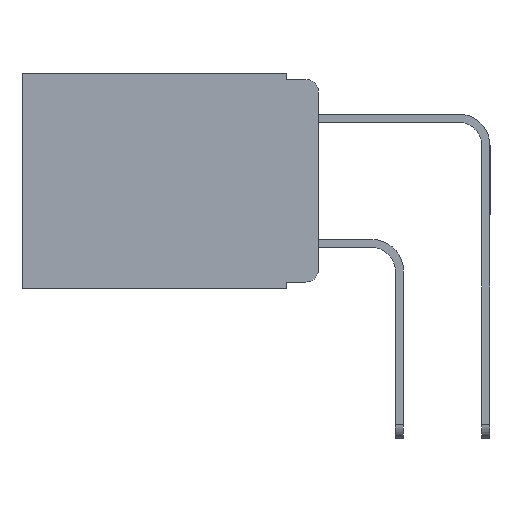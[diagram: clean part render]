
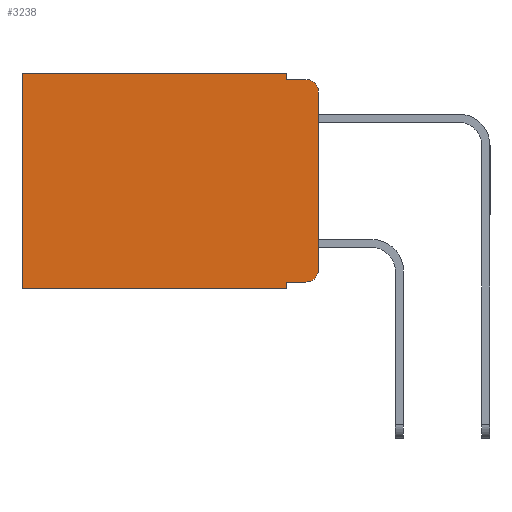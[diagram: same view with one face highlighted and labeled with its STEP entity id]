
A CAD part, left-side view. The second image highlights one B-rep face of the part: STEP entity #3238.
In plain terms, the highlighted planar face has unit normal (-1, 0, 0).
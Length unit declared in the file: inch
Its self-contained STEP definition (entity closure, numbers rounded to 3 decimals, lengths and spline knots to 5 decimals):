
#188 = ORIENTED_EDGE ( 'NONE', *, *, #21089, .T. ) ;
#479 = VECTOR ( 'NONE', #4422, 39.37008 ) ;
#505 = DIRECTION ( 'NONE',  ( 0., 0., -1. ) ) ;
#839 = DIRECTION ( 'NONE',  ( -1., 0., 0. ) ) ;
#938 = CARTESIAN_POINT ( 'NONE',  ( 0.298, 0.473, 0. ) ) ;
#1223 = CARTESIAN_POINT ( 'NONE',  ( 0.298, 0.051, 0. ) ) ;
#1309 = CARTESIAN_POINT ( 'NONE',  ( 0.298, 0.051, 0. ) ) ;
#1389 = CIRCLE ( 'NONE', #4869, 0.02 ) ;
#1470 = LINE ( 'NONE', #21075, #6059 ) ;
#1650 = LINE ( 'NONE', #11820, #15034 ) ;
#1971 = EDGE_CURVE ( 'NONE', #16292, #12738, #1470, .T. ) ;
#1996 = VERTEX_POINT ( 'NONE', #11594 ) ;
#2025 = VECTOR ( 'NONE', #15394, 39.37008 ) ;
#2137 = CARTESIAN_POINT ( 'NONE',  ( 0.298, 0.02, -0.01 ) ) ;
#2178 = CARTESIAN_POINT ( 'NONE',  ( 0.298, 0.051, 0. ) ) ;
#2614 = LINE ( 'NONE', #1223, #11169 ) ;
#2741 = ORIENTED_EDGE ( 'NONE', *, *, #18984, .F. ) ;
#2787 = DIRECTION ( 'NONE',  ( -1., 0., 0. ) ) ;
#2960 = DIRECTION ( 'NONE',  ( 0., 0., -1. ) ) ;
#3118 = DIRECTION ( 'NONE',  ( 0., 0., -1. ) ) ;
#3238 = ADVANCED_FACE ( 'NONE', ( #14812 ), #8622, .F. ) ;
#3830 = EDGE_CURVE ( 'NONE', #15052, #7431, #17042, .T. ) ;
#4422 = DIRECTION ( 'NONE',  ( 0., 0., -1. ) ) ;
#4861 = VERTEX_POINT ( 'NONE', #8842 ) ;
#4869 = AXIS2_PLACEMENT_3D ( 'NONE', #12919, #2787, #14503 ) ;
#5413 = CARTESIAN_POINT ( 'NONE',  ( 0.298, 0., 0. ) ) ;
#5426 = ORIENTED_EDGE ( 'NONE', *, *, #17950, .T. ) ;
#6059 = VECTOR ( 'NONE', #3118, 39.37008 ) ;
#6281 = CARTESIAN_POINT ( 'NONE',  ( 0.298, 0., -0.03 ) ) ;
#6320 = VERTEX_POINT ( 'NONE', #18817 ) ;
#7232 = DIRECTION ( 'NONE',  ( 0., 1., 0. ) ) ;
#7431 = VERTEX_POINT ( 'NONE', #15783 ) ;
#7881 = VERTEX_POINT ( 'NONE', #2137 ) ;
#7952 = VECTOR ( 'NONE', #17075, 39.37008 ) ;
#8490 = VERTEX_POINT ( 'NONE', #17010 ) ;
#8622 = PLANE ( 'NONE',  #13814 ) ;
#8842 = CARTESIAN_POINT ( 'NONE',  ( 0.298, 0.02, -0.333 ) ) ;
#8873 = ORIENTED_EDGE ( 'NONE', *, *, #16742, .T. ) ;
#9361 = ORIENTED_EDGE ( 'NONE', *, *, #14760, .T. ) ;
#10233 = CARTESIAN_POINT ( 'NONE',  ( 0.298, 0.051, -0.343 ) ) ;
#10744 = VECTOR ( 'NONE', #7232, 39.37008 ) ;
#11110 = CARTESIAN_POINT ( 'NONE',  ( 0.298, 0.02, -0.03 ) ) ;
#11169 = VECTOR ( 'NONE', #2960, 39.37008 ) ;
#11594 = CARTESIAN_POINT ( 'NONE',  ( 0.298, 0.473, 0. ) ) ;
#11820 = CARTESIAN_POINT ( 'NONE',  ( 0.298, 0.051, -0.333 ) ) ;
#11885 = DIRECTION ( 'NONE',  ( 0., 0., -1. ) ) ;
#12180 = CARTESIAN_POINT ( 'NONE',  ( 0.298, 0., -0.313 ) ) ;
#12728 = DIRECTION ( 'NONE',  ( 0., 0., -1. ) ) ;
#12738 = VERTEX_POINT ( 'NONE', #12180 ) ;
#12799 = AXIS2_PLACEMENT_3D ( 'NONE', #11110, #839, #12728 ) ;
#12919 = CARTESIAN_POINT ( 'NONE',  ( 0.298, 0.02, -0.313 ) ) ;
#13168 = VERTEX_POINT ( 'NONE', #1309 ) ;
#13460 = DIRECTION ( 'NONE',  ( 0., -1., 0. ) ) ;
#13665 = ORIENTED_EDGE ( 'NONE', *, *, #16870, .F. ) ;
#13798 = ORIENTED_EDGE ( 'NONE', *, *, #1971, .F. ) ;
#13814 = AXIS2_PLACEMENT_3D ( 'NONE', #19787, #21349, #11885 ) ;
#13897 = CARTESIAN_POINT ( 'NONE',  ( 0.298, 0., -0.343 ) ) ;
#13971 = LINE ( 'NONE', #938, #479 ) ;
#14183 = ORIENTED_EDGE ( 'NONE', *, *, #20027, .F. ) ;
#14503 = DIRECTION ( 'NONE',  ( 0., 0., -1. ) ) ;
#14760 = EDGE_CURVE ( 'NONE', #4861, #12738, #1389, .T. ) ;
#14812 = FACE_OUTER_BOUND ( 'NONE', #15744, .T. ) ;
#14907 = ORIENTED_EDGE ( 'NONE', *, *, #15793, .T. ) ;
#15034 = VECTOR ( 'NONE', #13460, 39.37008 ) ;
#15052 = VERTEX_POINT ( 'NONE', #10233 ) ;
#15394 = DIRECTION ( 'NONE',  ( 0., -1., 0. ) ) ;
#15744 = EDGE_LOOP ( 'NONE', ( #13798, #188, #14183, #2741, #8873, #5426, #20567, #13665, #14907, #9361 ) ) ;
#15783 = CARTESIAN_POINT ( 'NONE',  ( 0.298, 0.473, -0.343 ) ) ;
#15793 = EDGE_CURVE ( 'NONE', #6320, #4861, #1650, .T. ) ;
#16292 = VERTEX_POINT ( 'NONE', #6281 ) ;
#16718 = VECTOR ( 'NONE', #505, 39.37008 ) ;
#16742 = EDGE_CURVE ( 'NONE', #13168, #1996, #19194, .T. ) ;
#16870 = EDGE_CURVE ( 'NONE', #6320, #15052, #20901, .T. ) ;
#17010 = CARTESIAN_POINT ( 'NONE',  ( 0.298, 0.051, -0.01 ) ) ;
#17042 = LINE ( 'NONE', #13897, #7952 ) ;
#17075 = DIRECTION ( 'NONE',  ( 0., 1., 0. ) ) ;
#17950 = EDGE_CURVE ( 'NONE', #1996, #7431, #13971, .T. ) ;
#18065 = CIRCLE ( 'NONE', #12799, 0.02 ) ;
#18573 = CARTESIAN_POINT ( 'NONE',  ( 0.298, 0.051, -0.01 ) ) ;
#18817 = CARTESIAN_POINT ( 'NONE',  ( 0.298, 0.051, -0.333 ) ) ;
#18984 = EDGE_CURVE ( 'NONE', #13168, #8490, #2614, .T. ) ;
#19194 = LINE ( 'NONE', #5413, #10744 ) ;
#19787 = CARTESIAN_POINT ( 'NONE',  ( 0.298, 0., 0. ) ) ;
#20027 = EDGE_CURVE ( 'NONE', #8490, #7881, #20045, .T. ) ;
#20045 = LINE ( 'NONE', #18573, #2025 ) ;
#20567 = ORIENTED_EDGE ( 'NONE', *, *, #3830, .F. ) ;
#20901 = LINE ( 'NONE', #2178, #16718 ) ;
#21075 = CARTESIAN_POINT ( 'NONE',  ( 0.298, 0., 0. ) ) ;
#21089 = EDGE_CURVE ( 'NONE', #16292, #7881, #18065, .T. ) ;
#21349 = DIRECTION ( 'NONE',  ( 1., 0., 0. ) ) ;
